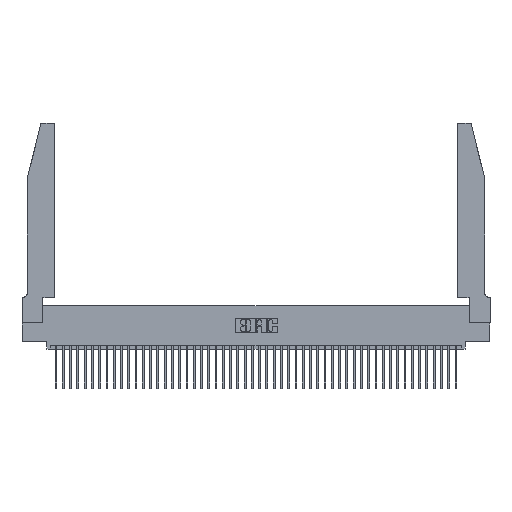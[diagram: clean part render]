
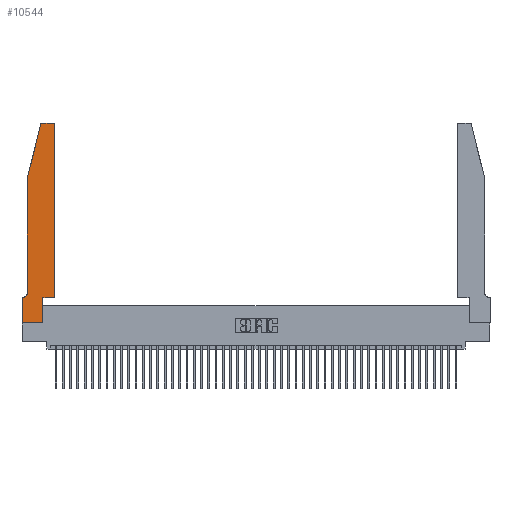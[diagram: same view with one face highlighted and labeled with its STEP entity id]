
A CAD part, top view. The second image highlights one B-rep face of the part: STEP entity #10544.
In plain terms, the highlighted planar face has unit normal (0, 0, 1).
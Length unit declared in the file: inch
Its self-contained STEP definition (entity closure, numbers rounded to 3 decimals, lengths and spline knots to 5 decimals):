
#545 = LINE ( 'NONE', #29126, #8017 ) ;
#977 = CARTESIAN_POINT ( 'NONE',  ( 0.2605, 2.75, 0.37 ) ) ;
#1106 = DIRECTION ( 'NONE',  ( 0., 0., -1. ) ) ;
#4199 = DIRECTION ( 'NONE',  ( -1., 0., 0. ) ) ;
#4343 = DIRECTION ( 'NONE',  ( 0., 0., 1. ) ) ;
#4530 = CARTESIAN_POINT ( 'NONE',  ( 0., 0., 0.37 ) ) ;
#5179 = CARTESIAN_POINT ( 'NONE',  ( 0.2865, 0.35, 0.37 ) ) ;
#5895 = DIRECTION ( 'NONE',  ( 0., 1., 0. ) ) ;
#5903 = CARTESIAN_POINT ( 'NONE',  ( 0.0755, 0.42, 0.37 ) ) ;
#5995 = CARTESIAN_POINT ( 'NONE',  ( 0.0755, 2., 0.37 ) ) ;
#6069 = DIRECTION ( 'NONE',  ( 1., 0., 0. ) ) ;
#6512 = LINE ( 'NONE', #36829, #43894 ) ;
#6733 = DIRECTION ( 'NONE',  ( 0., 0., 1. ) ) ;
#6762 = AXIS2_PLACEMENT_3D ( 'NONE', #37445, #1106, #15420 ) ;
#7769 = VERTEX_POINT ( 'NONE', #11463 ) ;
#7938 = VECTOR ( 'NONE', #23836, 39.37008 ) ;
#8017 = VECTOR ( 'NONE', #22927, 39.37008 ) ;
#8268 = CARTESIAN_POINT ( 'NONE',  ( 0.284, 2.75, 0.37 ) ) ;
#8535 = LINE ( 'NONE', #13079, #7938 ) ;
#10295 = VERTEX_POINT ( 'NONE', #5903 ) ;
#10544 = ADVANCED_FACE ( 'NONE', ( #35340 ), #43934, .T. ) ;
#10833 = VERTEX_POINT ( 'NONE', #45895 ) ;
#11325 = CARTESIAN_POINT ( 'NONE',  ( 0.2865, 0., 0.37 ) ) ;
#11463 = CARTESIAN_POINT ( 'NONE',  ( 0., 0.35, 0.37 ) ) ;
#11505 = LINE ( 'NONE', #5179, #43237 ) ;
#12470 = EDGE_CURVE ( 'NONE', #10833, #32101, #19810, .T. ) ;
#13063 = ORIENTED_EDGE ( 'NONE', *, *, #22802, .T. ) ;
#13079 = CARTESIAN_POINT ( 'NONE',  ( 0.4505, 0.35, 0.37 ) ) ;
#15074 = DIRECTION ( 'NONE',  ( -0.239, -0.971, 0. ) ) ;
#15420 = DIRECTION ( 'NONE',  ( -1., 0., 0. ) ) ;
#15776 = AXIS2_PLACEMENT_3D ( 'NONE', #42381, #6733, #27943 ) ;
#16734 = EDGE_CURVE ( 'NONE', #34612, #40388, #33205, .T. ) ;
#17105 = ORIENTED_EDGE ( 'NONE', *, *, #28626, .T. ) ;
#17913 = VERTEX_POINT ( 'NONE', #35099 ) ;
#18469 = VERTEX_POINT ( 'NONE', #40834 ) ;
#18859 = ORIENTED_EDGE ( 'NONE', *, *, #30821, .T. ) ;
#19024 = EDGE_CURVE ( 'NONE', #40388, #18469, #11505, .T. ) ;
#19810 = LINE ( 'NONE', #977, #39592 ) ;
#20866 = VERTEX_POINT ( 'NONE', #22459 ) ;
#20868 = CARTESIAN_POINT ( 'NONE',  ( 0., 0., 0.37 ) ) ;
#21865 = CIRCLE ( 'NONE', #15776, 0.03 ) ;
#21923 = DIRECTION ( 'NONE',  ( 1., 0., 0. ) ) ;
#21933 = EDGE_LOOP ( 'NONE', ( #26587, #24826, #23997, #42953, #17105, #13063, #35244, #24957, #24698, #18859, #23888, #22823 ) ) ;
#22459 = CARTESIAN_POINT ( 'NONE',  ( 0.25487, 2.72718, 0.37 ) ) ;
#22802 = EDGE_CURVE ( 'NONE', #17913, #7769, #26481, .T. ) ;
#22823 = ORIENTED_EDGE ( 'NONE', *, *, #37329, .T. ) ;
#22927 = DIRECTION ( 'NONE',  ( 0., -1., 0. ) ) ;
#23533 = LINE ( 'NONE', #4530, #41119 ) ;
#23836 = DIRECTION ( 'NONE',  ( 1., 0., 0. ) ) ;
#23888 = ORIENTED_EDGE ( 'NONE', *, *, #37130, .T. ) ;
#23997 = ORIENTED_EDGE ( 'NONE', *, *, #34780, .T. ) ;
#24698 = ORIENTED_EDGE ( 'NONE', *, *, #19024, .T. ) ;
#24826 = ORIENTED_EDGE ( 'NONE', *, *, #39645, .T. ) ;
#24957 = ORIENTED_EDGE ( 'NONE', *, *, #16734, .T. ) ;
#25080 = DIRECTION ( 'NONE',  ( 0., 0., 1. ) ) ;
#26107 = EDGE_CURVE ( 'NONE', #32793, #10295, #545, .T. ) ;
#26481 = LINE ( 'NONE', #40270, #45243 ) ;
#26587 = ORIENTED_EDGE ( 'NONE', *, *, #12470, .T. ) ;
#27692 = VECTOR ( 'NONE', #5895, 39.37008 ) ;
#27943 = DIRECTION ( 'NONE',  ( 1., 0., 0. ) ) ;
#28626 = EDGE_CURVE ( 'NONE', #10295, #17913, #46474, .T. ) ;
#29126 = CARTESIAN_POINT ( 'NONE',  ( 0.0755, 2., 0.37 ) ) ;
#30284 = CARTESIAN_POINT ( 'NONE',  ( 0.4505, 2.72, 0.37 ) ) ;
#30507 = DIRECTION ( 'NONE',  ( -1., 0., 0. ) ) ;
#30821 = EDGE_CURVE ( 'NONE', #18469, #37191, #8535, .T. ) ;
#32101 = VERTEX_POINT ( 'NONE', #8268 ) ;
#32793 = VERTEX_POINT ( 'NONE', #5995 ) ;
#33062 = AXIS2_PLACEMENT_3D ( 'NONE', #37280, #4343, #37907 ) ;
#33205 = LINE ( 'NONE', #20868, #36093 ) ;
#34407 = EDGE_CURVE ( 'NONE', #7769, #34612, #23533, .T. ) ;
#34612 = VERTEX_POINT ( 'NONE', #42366 ) ;
#34780 = EDGE_CURVE ( 'NONE', #20866, #32793, #6512, .T. ) ;
#34976 = VERTEX_POINT ( 'NONE', #30284 ) ;
#35064 = CARTESIAN_POINT ( 'NONE',  ( 0.4505, 0.35, 0.37 ) ) ;
#35099 = CARTESIAN_POINT ( 'NONE',  ( 0.0055, 0.35, 0.37 ) ) ;
#35244 = ORIENTED_EDGE ( 'NONE', *, *, #34407, .T. ) ;
#35340 = FACE_OUTER_BOUND ( 'NONE', #21933, .T. ) ;
#36093 = VECTOR ( 'NONE', #6069, 39.37008 ) ;
#36829 = CARTESIAN_POINT ( 'NONE',  ( 0.0755, 2., 0.37 ) ) ;
#37130 = EDGE_CURVE ( 'NONE', #37191, #34976, #37324, .T. ) ;
#37191 = VERTEX_POINT ( 'NONE', #35064 ) ;
#37280 = CARTESIAN_POINT ( 'NONE',  ( 0., 0.35, 0.37 ) ) ;
#37324 = LINE ( 'NONE', #42322, #27692 ) ;
#37329 = EDGE_CURVE ( 'NONE', #34976, #10833, #38436, .T. ) ;
#37445 = CARTESIAN_POINT ( 'NONE',  ( 0.0055, 0.42, 0.37 ) ) ;
#37907 = DIRECTION ( 'NONE',  ( 1., 0., 0. ) ) ;
#37938 = CARTESIAN_POINT ( 'NONE',  ( 0.4205, 2.72, 0.37 ) ) ;
#38436 = CIRCLE ( 'NONE', #46098, 0.03 ) ;
#39592 = VECTOR ( 'NONE', #30507, 39.37008 ) ;
#39645 = EDGE_CURVE ( 'NONE', #32101, #20866, #21865, .T. ) ;
#40270 = CARTESIAN_POINT ( 'NONE',  ( 0.0755, 0.35, 0.37 ) ) ;
#40388 = VERTEX_POINT ( 'NONE', #11325 ) ;
#40834 = CARTESIAN_POINT ( 'NONE',  ( 0.2865, 0.35, 0.37 ) ) ;
#41119 = VECTOR ( 'NONE', #44419, 39.37008 ) ;
#41941 = DIRECTION ( 'NONE',  ( 0., 1., 0. ) ) ;
#42322 = CARTESIAN_POINT ( 'NONE',  ( 0.4505, 0.35, 0.37 ) ) ;
#42366 = CARTESIAN_POINT ( 'NONE',  ( 0., 0., 0.37 ) ) ;
#42381 = CARTESIAN_POINT ( 'NONE',  ( 0.284, 2.72, 0.37 ) ) ;
#42953 = ORIENTED_EDGE ( 'NONE', *, *, #26107, .T. ) ;
#43237 = VECTOR ( 'NONE', #41941, 39.37008 ) ;
#43894 = VECTOR ( 'NONE', #15074, 39.37008 ) ;
#43934 = PLANE ( 'NONE',  #33062 ) ;
#44419 = DIRECTION ( 'NONE',  ( 0., -1., 0. ) ) ;
#45243 = VECTOR ( 'NONE', #4199, 39.37008 ) ;
#45895 = CARTESIAN_POINT ( 'NONE',  ( 0.4205, 2.75, 0.37 ) ) ;
#46098 = AXIS2_PLACEMENT_3D ( 'NONE', #37938, #25080, #21923 ) ;
#46474 = CIRCLE ( 'NONE', #6762, 0.07 ) ;
